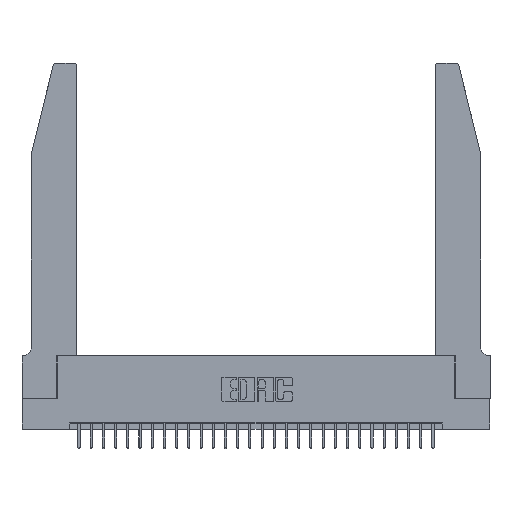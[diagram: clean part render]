
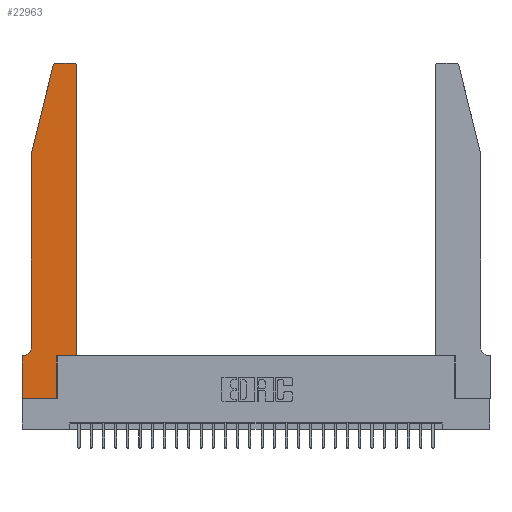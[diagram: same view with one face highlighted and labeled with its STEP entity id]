
A CAD part, top view. The second image highlights one B-rep face of the part: STEP entity #22963.
In plain terms, the highlighted planar face has unit normal (0, 0, 1).
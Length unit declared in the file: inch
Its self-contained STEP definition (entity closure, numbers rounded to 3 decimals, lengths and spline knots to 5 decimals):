
#42 = CARTESIAN_POINT ( 'NONE',  ( 0., 0.35, 0.37 ) ) ;
#358 = EDGE_CURVE ( 'NONE', #8783, #2497, #15418, .T. ) ;
#476 = AXIS2_PLACEMENT_3D ( 'NONE', #14861, #23987, #929 ) ;
#929 = DIRECTION ( 'NONE',  ( 1., 0., 0. ) ) ;
#1000 = LINE ( 'NONE', #16173, #16531 ) ;
#1210 = CARTESIAN_POINT ( 'NONE',  ( 0.0055, 0.35, 0.37 ) ) ;
#1329 = LINE ( 'NONE', #4795, #2390 ) ;
#1590 = LINE ( 'NONE', #7028, #18265 ) ;
#1670 = LINE ( 'NONE', #25113, #28780 ) ;
#1689 = DIRECTION ( 'NONE',  ( 1., 0., 0. ) ) ;
#1719 = CARTESIAN_POINT ( 'NONE',  ( 0.0755, 2., 0.37 ) ) ;
#1771 = EDGE_CURVE ( 'NONE', #14802, #21567, #1590, .T. ) ;
#2291 = DIRECTION ( 'NONE',  ( -1., 0., 0. ) ) ;
#2348 = CARTESIAN_POINT ( 'NONE',  ( 0.0755, 2., 0.37 ) ) ;
#2390 = VECTOR ( 'NONE', #21256, 39.37008 ) ;
#2408 = EDGE_CURVE ( 'NONE', #3148, #7040, #1670, .T. ) ;
#2465 = ORIENTED_EDGE ( 'NONE', *, *, #2408, .T. ) ;
#2497 = VERTEX_POINT ( 'NONE', #1719 ) ;
#2611 = ORIENTED_EDGE ( 'NONE', *, *, #5016, .T. ) ;
#2678 = EDGE_LOOP ( 'NONE', ( #2611, #17260, #24900, #4399, #21455, #28320, #13915, #5708, #23851, #16320, #2465, #23390 ) ) ;
#2850 = FACE_OUTER_BOUND ( 'NONE', #2678, .T. ) ;
#3148 = VERTEX_POINT ( 'NONE', #24219 ) ;
#4234 = VECTOR ( 'NONE', #2291, 39.37008 ) ;
#4399 = ORIENTED_EDGE ( 'NONE', *, *, #17793, .T. ) ;
#4795 = CARTESIAN_POINT ( 'NONE',  ( 0.4505, 0.35, 0.37 ) ) ;
#5016 = EDGE_CURVE ( 'NONE', #19272, #8957, #27803, .T. ) ;
#5708 = ORIENTED_EDGE ( 'NONE', *, *, #19704, .T. ) ;
#6690 = DIRECTION ( 'NONE',  ( -1., 0., 0. ) ) ;
#6749 = CARTESIAN_POINT ( 'NONE',  ( 0.4205, 2.75, 0.37 ) ) ;
#7028 = CARTESIAN_POINT ( 'NONE',  ( 0., 0., 0.37 ) ) ;
#7040 = VERTEX_POINT ( 'NONE', #19865 ) ;
#7508 = DIRECTION ( 'NONE',  ( 1., 0., 0. ) ) ;
#7536 = CARTESIAN_POINT ( 'NONE',  ( 0.0755, 0.35, 0.37 ) ) ;
#8093 = CARTESIAN_POINT ( 'NONE',  ( 0.25487, 2.72718, 0.37 ) ) ;
#8204 = CARTESIAN_POINT ( 'NONE',  ( 0.2865, 0., 0.37 ) ) ;
#8305 = DIRECTION ( 'NONE',  ( 1., 0., 0. ) ) ;
#8534 = VECTOR ( 'NONE', #25278, 39.37008 ) ;
#8637 = AXIS2_PLACEMENT_3D ( 'NONE', #25032, #20569, #6690 ) ;
#8783 = VERTEX_POINT ( 'NONE', #8093 ) ;
#8957 = VERTEX_POINT ( 'NONE', #23291 ) ;
#9847 = VERTEX_POINT ( 'NONE', #1210 ) ;
#9945 = EDGE_CURVE ( 'NONE', #7040, #19272, #21741, .T. ) ;
#9985 = VECTOR ( 'NONE', #26078, 39.37008 ) ;
#12027 = EDGE_CURVE ( 'NONE', #29879, #9847, #25286, .T. ) ;
#12058 = DIRECTION ( 'NONE',  ( 0., 0., 1. ) ) ;
#12195 = EDGE_CURVE ( 'NONE', #25639, #15573, #1000, .T. ) ;
#13138 = EDGE_CURVE ( 'NONE', #9847, #14802, #21211, .T. ) ;
#13523 = DIRECTION ( 'NONE',  ( 0., 1., 0. ) ) ;
#13600 = CARTESIAN_POINT ( 'NONE',  ( 0.0755, 2., 0.37 ) ) ;
#13915 = ORIENTED_EDGE ( 'NONE', *, *, #1771, .T. ) ;
#14110 = VECTOR ( 'NONE', #16377, 39.37008 ) ;
#14140 = EDGE_CURVE ( 'NONE', #8957, #8783, #14261, .T. ) ;
#14261 = CIRCLE ( 'NONE', #15074, 0.03 ) ;
#14802 = VERTEX_POINT ( 'NONE', #42 ) ;
#14861 = CARTESIAN_POINT ( 'NONE',  ( 0., 0.35, 0.37 ) ) ;
#14992 = DIRECTION ( 'NONE',  ( 0., 0., 1. ) ) ;
#15074 = AXIS2_PLACEMENT_3D ( 'NONE', #21980, #14992, #8305 ) ;
#15418 = LINE ( 'NONE', #13600, #8534 ) ;
#15573 = VERTEX_POINT ( 'NONE', #23484 ) ;
#15764 = CARTESIAN_POINT ( 'NONE',  ( 0.0755, 0.42, 0.37 ) ) ;
#16166 = DIRECTION ( 'NONE',  ( 0., -1., 0. ) ) ;
#16173 = CARTESIAN_POINT ( 'NONE',  ( 0.2865, 0.35, 0.37 ) ) ;
#16320 = ORIENTED_EDGE ( 'NONE', *, *, #20015, .T. ) ;
#16377 = DIRECTION ( 'NONE',  ( 0., -1., 0. ) ) ;
#16464 = CARTESIAN_POINT ( 'NONE',  ( 0., 0., 0.37 ) ) ;
#16531 = VECTOR ( 'NONE', #13523, 39.37008 ) ;
#17260 = ORIENTED_EDGE ( 'NONE', *, *, #14140, .T. ) ;
#17793 = EDGE_CURVE ( 'NONE', #2497, #29879, #26059, .T. ) ;
#18265 = VECTOR ( 'NONE', #16166, 39.37008 ) ;
#19272 = VERTEX_POINT ( 'NONE', #6749 ) ;
#19704 = EDGE_CURVE ( 'NONE', #21567, #25639, #20877, .T. ) ;
#19865 = CARTESIAN_POINT ( 'NONE',  ( 0.4505, 2.72, 0.37 ) ) ;
#20015 = EDGE_CURVE ( 'NONE', #15573, #3148, #1329, .T. ) ;
#20525 = VECTOR ( 'NONE', #1689, 39.37008 ) ;
#20569 = DIRECTION ( 'NONE',  ( 0., 0., -1. ) ) ;
#20877 = LINE ( 'NONE', #29216, #20525 ) ;
#21211 = LINE ( 'NONE', #7536, #9985 ) ;
#21256 = DIRECTION ( 'NONE',  ( 1., 0., 0. ) ) ;
#21455 = ORIENTED_EDGE ( 'NONE', *, *, #12027, .T. ) ;
#21567 = VERTEX_POINT ( 'NONE', #16464 ) ;
#21741 = CIRCLE ( 'NONE', #25471, 0.03 ) ;
#21856 = PLANE ( 'NONE',  #476 ) ;
#21980 = CARTESIAN_POINT ( 'NONE',  ( 0.284, 2.72, 0.37 ) ) ;
#22963 = ADVANCED_FACE ( 'NONE', ( #2850 ), #21856, .T. ) ;
#23291 = CARTESIAN_POINT ( 'NONE',  ( 0.284, 2.75, 0.37 ) ) ;
#23390 = ORIENTED_EDGE ( 'NONE', *, *, #9945, .T. ) ;
#23484 = CARTESIAN_POINT ( 'NONE',  ( 0.2865, 0.35, 0.37 ) ) ;
#23851 = ORIENTED_EDGE ( 'NONE', *, *, #12195, .T. ) ;
#23987 = DIRECTION ( 'NONE',  ( 0., 0., 1. ) ) ;
#24219 = CARTESIAN_POINT ( 'NONE',  ( 0.4505, 0.35, 0.37 ) ) ;
#24348 = DIRECTION ( 'NONE',  ( 0., 1., 0. ) ) ;
#24900 = ORIENTED_EDGE ( 'NONE', *, *, #358, .T. ) ;
#25032 = CARTESIAN_POINT ( 'NONE',  ( 0.0055, 0.42, 0.37 ) ) ;
#25113 = CARTESIAN_POINT ( 'NONE',  ( 0.4505, 0.35, 0.37 ) ) ;
#25278 = DIRECTION ( 'NONE',  ( -0.239, -0.971, 0. ) ) ;
#25286 = CIRCLE ( 'NONE', #8637, 0.07 ) ;
#25471 = AXIS2_PLACEMENT_3D ( 'NONE', #25952, #12058, #7508 ) ;
#25639 = VERTEX_POINT ( 'NONE', #8204 ) ;
#25952 = CARTESIAN_POINT ( 'NONE',  ( 0.4205, 2.72, 0.37 ) ) ;
#26059 = LINE ( 'NONE', #2348, #14110 ) ;
#26078 = DIRECTION ( 'NONE',  ( -1., 0., 0. ) ) ;
#27500 = CARTESIAN_POINT ( 'NONE',  ( 0.2605, 2.75, 0.37 ) ) ;
#27803 = LINE ( 'NONE', #27500, #4234 ) ;
#28320 = ORIENTED_EDGE ( 'NONE', *, *, #13138, .T. ) ;
#28780 = VECTOR ( 'NONE', #24348, 39.37008 ) ;
#29216 = CARTESIAN_POINT ( 'NONE',  ( 0., 0., 0.37 ) ) ;
#29879 = VERTEX_POINT ( 'NONE', #15764 ) ;
